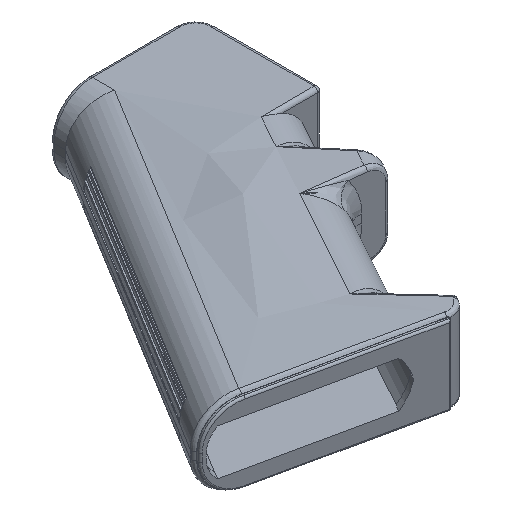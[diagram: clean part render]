
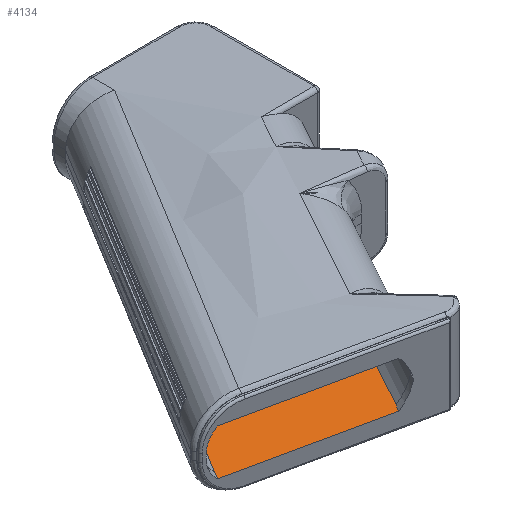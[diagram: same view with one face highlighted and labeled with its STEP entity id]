
A CAD part, isometric view. The second image highlights one B-rep face of the part: STEP entity #4134.
In plain terms, the highlighted planar face has unit normal (0, 0, 1).
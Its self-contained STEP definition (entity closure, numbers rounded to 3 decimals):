
#56 = PLANE ( 'NONE',  #7434 ) ;
#94 = CARTESIAN_POINT ( 'NONE',  ( -217.737, -118.423, -6.263 ) ) ;
#129 = LINE ( 'NONE', #1884, #4485 ) ;
#262 = CARTESIAN_POINT ( 'NONE',  ( -169.926, -40.28, -6.263 ) ) ;
#361 = VECTOR ( 'NONE', #5247, 1000. ) ;
#647 = EDGE_CURVE ( 'NONE', #1714, #5473, #5894, .T. ) ;
#969 = DIRECTION ( 'NONE',  ( 0.865, -0.502, 0. ) ) ;
#1009 = VECTOR ( 'NONE', #6203, 1000. ) ;
#1156 = ORIENTED_EDGE ( 'NONE', *, *, #4772, .F. ) ;
#1434 = CARTESIAN_POINT ( 'NONE',  ( -140.39, -57.411, -6.263 ) ) ;
#1520 = CARTESIAN_POINT ( 'NONE',  ( -177.638, -125.009, -6.262 ) ) ;
#1559 = FACE_OUTER_BOUND ( 'NONE', #3894, .T. ) ;
#1714 = VERTEX_POINT ( 'NONE', #1520 ) ;
#1884 = CARTESIAN_POINT ( 'NONE',  ( -218.671, -118.222, -6.263 ) ) ;
#2030 = CARTESIAN_POINT ( 'NONE',  ( -181.461, -131.6, -6.262 ) ) ;
#2123 = ORIENTED_EDGE ( 'NONE', *, *, #7164, .F. ) ;
#2198 = DIRECTION ( 'NONE',  ( -1., 0., 0. ) ) ;
#2216 = LINE ( 'NONE', #262, #7386 ) ;
#2349 = CARTESIAN_POINT ( 'NONE',  ( -220.505, -123.196, -6.263 ) ) ;
#2484 = VERTEX_POINT ( 'NONE', #7648 ) ;
#2594 = ORIENTED_EDGE ( 'NONE', *, *, #4359, .F. ) ;
#2597 = DIRECTION ( 'NONE',  ( 0.978, -0.21, 0. ) ) ;
#2755 = EDGE_CURVE ( 'NONE', #8118, #6839, #129, .T. ) ;
#3058 = DIRECTION ( 'NONE',  ( 0.502, 0.865, 0. ) ) ;
#3186 = CARTESIAN_POINT ( 'NONE',  ( -216.682, -116.605, -6.263 ) ) ;
#3226 = CARTESIAN_POINT ( 'NONE',  ( -169.926, -40.28, -6.263 ) ) ;
#3251 = ORIENTED_EDGE ( 'NONE', *, *, #4648, .T. ) ;
#3854 = VECTOR ( 'NONE', #3058, 1000. ) ;
#3894 = EDGE_LOOP ( 'NONE', ( #2594, #1156, #7225, #3251, #5865, #2123 ) ) ;
#4134 = ADVANCED_FACE ( 'NONE', ( #1559 ), #56, .F. ) ;
#4359 = EDGE_CURVE ( 'NONE', #2484, #5302, #7876, .T. ) ;
#4485 = VECTOR ( 'NONE', #2597, 1000. ) ;
#4648 = EDGE_CURVE ( 'NONE', #6839, #1714, #6524, .T. ) ;
#4772 = EDGE_CURVE ( 'NONE', #8118, #2484, #6314, .T. ) ;
#4941 = CARTESIAN_POINT ( 'NONE',  ( -217.697, -39.766, -6.263 ) ) ;
#5247 = DIRECTION ( 'NONE',  ( 0.483, 0.876, 0. ) ) ;
#5302 = VERTEX_POINT ( 'NONE', #3226 ) ;
#5473 = VERTEX_POINT ( 'NONE', #1434 ) ;
#5865 = ORIENTED_EDGE ( 'NONE', *, *, #647, .T. ) ;
#5894 = LINE ( 'NONE', #7176, #361 ) ;
#6203 = DIRECTION ( 'NONE',  ( 0.502, 0.865, 0. ) ) ;
#6314 = LINE ( 'NONE', #2349, #3854 ) ;
#6330 = DIRECTION ( 'NONE',  ( 0., 0., -1. ) ) ;
#6425 = VECTOR ( 'NONE', #7826, 1000. ) ;
#6524 = LINE ( 'NONE', #2030, #1009 ) ;
#6839 = VERTEX_POINT ( 'NONE', #8385 ) ;
#7164 = EDGE_CURVE ( 'NONE', #5302, #5473, #2216, .T. ) ;
#7176 = CARTESIAN_POINT ( 'NONE',  ( -177.638, -125.009, -6.263 ) ) ;
#7225 = ORIENTED_EDGE ( 'NONE', *, *, #2755, .T. ) ;
#7386 = VECTOR ( 'NONE', #969, 1000. ) ;
#7434 = AXIS2_PLACEMENT_3D ( 'NONE', #4941, #6330, #2198 ) ;
#7648 = CARTESIAN_POINT ( 'NONE',  ( -216.682, -116.605, -6.263 ) ) ;
#7826 = DIRECTION ( 'NONE',  ( 0.522, 0.853, 0. ) ) ;
#7876 = LINE ( 'NONE', #3186, #6425 ) ;
#8118 = VERTEX_POINT ( 'NONE', #94 ) ;
#8385 = CARTESIAN_POINT ( 'NONE',  ( -178.693, -126.828, -6.262 ) ) ;
